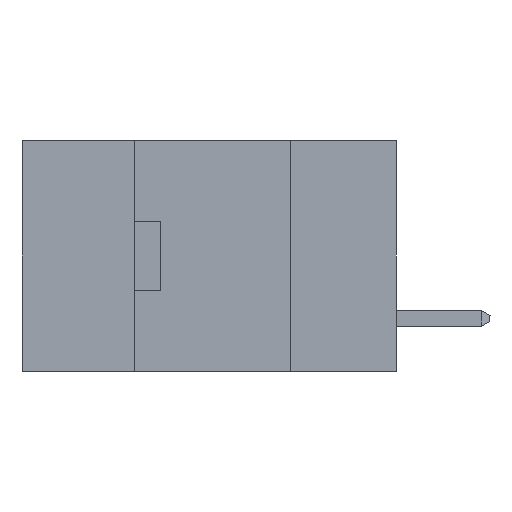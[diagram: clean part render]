
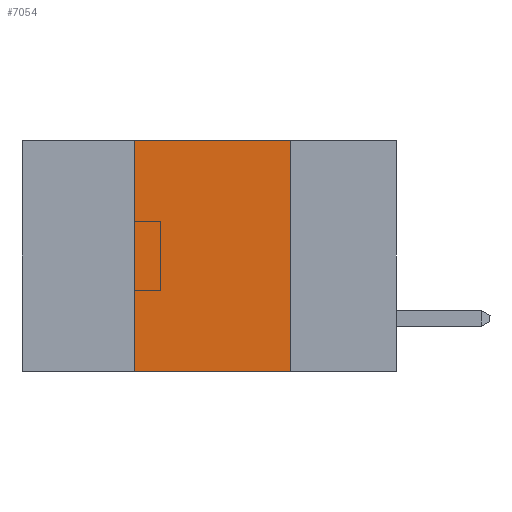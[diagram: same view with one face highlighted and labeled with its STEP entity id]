
A CAD part, left-side view. The second image highlights one B-rep face of the part: STEP entity #7054.
In plain terms, the highlighted planar face has unit normal (-1, 0, 0).
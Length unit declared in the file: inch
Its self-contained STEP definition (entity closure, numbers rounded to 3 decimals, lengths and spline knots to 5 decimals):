
#2 = CARTESIAN_POINT ( 'NONE',  ( 0., 0.42, -0.37 ) ) ;
#1160 = VERTEX_POINT ( 'NONE', #24381 ) ;
#1217 = EDGE_LOOP ( 'NONE', ( #11638, #20627, #22531, #4749 ) ) ;
#1309 = CARTESIAN_POINT ( 'NONE',  ( 0., 0.6, -0.37 ) ) ;
#2107 = DIRECTION ( 'NONE',  ( 0., 0., 1. ) ) ;
#3041 = CARTESIAN_POINT ( 'NONE',  ( 0., 0.17, -0.37 ) ) ;
#3129 = EDGE_CURVE ( 'NONE', #10644, #7369, #14650, .T. ) ;
#3154 = VECTOR ( 'NONE', #3612, 39.37008 ) ;
#3542 = CARTESIAN_POINT ( 'NONE',  ( 0., 0.17, 0. ) ) ;
#3612 = DIRECTION ( 'NONE',  ( 0., -1., 0. ) ) ;
#3775 = AXIS2_PLACEMENT_3D ( 'NONE', #21792, #23979, #11498 ) ;
#4749 = ORIENTED_EDGE ( 'NONE', *, *, #6411, .T. ) ;
#5237 = FACE_OUTER_BOUND ( 'NONE', #1217, .T. ) ;
#5860 = LINE ( 'NONE', #1309, #23134 ) ;
#6411 = EDGE_CURVE ( 'NONE', #1160, #7369, #5860, .T. ) ;
#7054 = ADVANCED_FACE ( 'NONE', ( #5237 ), #9398, .F. ) ;
#7369 = VERTEX_POINT ( 'NONE', #20723 ) ;
#7810 = CARTESIAN_POINT ( 'NONE',  ( 0., 0.6, 0. ) ) ;
#9398 = PLANE ( 'NONE',  #3775 ) ;
#9793 = EDGE_CURVE ( 'NONE', #22324, #10644, #19785, .T. ) ;
#9990 = LINE ( 'NONE', #2, #25331 ) ;
#10644 = VERTEX_POINT ( 'NONE', #3542 ) ;
#11498 = DIRECTION ( 'NONE',  ( 0., 0., -1. ) ) ;
#11638 = ORIENTED_EDGE ( 'NONE', *, *, #3129, .F. ) ;
#14650 = LINE ( 'NONE', #3041, #15970 ) ;
#15777 = CARTESIAN_POINT ( 'NONE',  ( 0., 0.42, 0. ) ) ;
#15970 = VECTOR ( 'NONE', #23907, 39.37008 ) ;
#17995 = DIRECTION ( 'NONE',  ( 0., -1., 0. ) ) ;
#19785 = LINE ( 'NONE', #7810, #3154 ) ;
#20627 = ORIENTED_EDGE ( 'NONE', *, *, #9793, .F. ) ;
#20723 = CARTESIAN_POINT ( 'NONE',  ( 0., 0.17, -0.37 ) ) ;
#21792 = CARTESIAN_POINT ( 'NONE',  ( 0., 0.6, 0. ) ) ;
#22324 = VERTEX_POINT ( 'NONE', #15777 ) ;
#22531 = ORIENTED_EDGE ( 'NONE', *, *, #22606, .F. ) ;
#22606 = EDGE_CURVE ( 'NONE', #1160, #22324, #9990, .T. ) ;
#23134 = VECTOR ( 'NONE', #17995, 39.37008 ) ;
#23907 = DIRECTION ( 'NONE',  ( 0., 0., -1. ) ) ;
#23979 = DIRECTION ( 'NONE',  ( 1., 0., 0. ) ) ;
#24381 = CARTESIAN_POINT ( 'NONE',  ( 0., 0.42, -0.37 ) ) ;
#25331 = VECTOR ( 'NONE', #2107, 39.37008 ) ;
